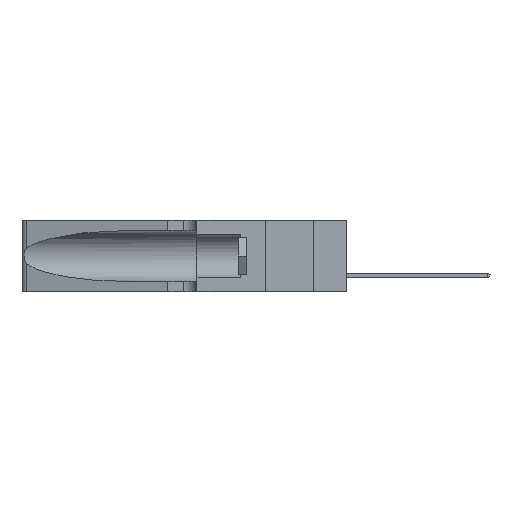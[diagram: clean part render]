
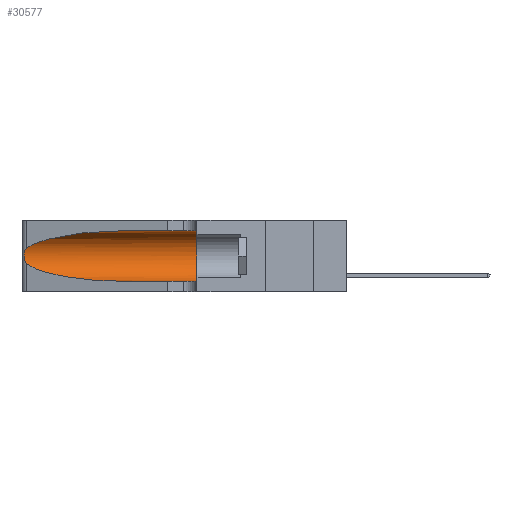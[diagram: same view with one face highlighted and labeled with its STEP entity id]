
A CAD part, left-side view. The second image highlights one B-rep face of the part: STEP entity #30577.
In plain terms, the highlighted cylindrical face has radius 3.308 mm (diameter 6.617 mm), a partial arc.
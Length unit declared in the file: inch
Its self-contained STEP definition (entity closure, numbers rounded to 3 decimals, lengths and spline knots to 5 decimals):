
#126 = CARTESIAN_POINT ( 'NONE',  ( 0.2373, 1.15595, 0.28018 ) ) ;
#372 = VERTEX_POINT ( 'NONE', #4743 ) ;
#476 = CARTESIAN_POINT ( 'NONE',  ( 0.1305, 1.61858, 0.05475 ) ) ;
#1925 = EDGE_CURVE ( 'NONE', #12517, #10170, #16900, .T. ) ;
#2455 = CARTESIAN_POINT ( 'NONE',  ( 0.18966, 0.96281, 0.31525 ) ) ;
#2658 = CARTESIAN_POINT ( 'NONE',  ( 0.25487, 1.22718, 0.22369 ) ) ;
#3737 = CARTESIAN_POINT ( 'NONE',  ( 0.25639, 1.23186, 0.15144 ) ) ;
#4407 = DIRECTION ( 'NONE',  ( 0., -1., 0. ) ) ;
#4561 = CARTESIAN_POINT ( 'NONE',  ( 0.1305, 0.72297, 0.05475 ) ) ;
#4666 = CARTESIAN_POINT ( 'NONE',  ( 0.2373, 1.15595, 0.08982 ) ) ;
#4743 = CARTESIAN_POINT ( 'NONE',  ( 0.1305, 0.72297, 0.05475 ) ) ;
#5673 = CARTESIAN_POINT ( 'NONE',  ( 0.1305, 0.35, 0.31525 ) ) ;
#6467 = CARTESIAN_POINT ( 'NONE',  ( 0.25787, 1.23484, 0.2124 ) ) ;
#6746 = CARTESIAN_POINT ( 'NONE',  ( 0.25487, 1.22718, 0.14631 ) ) ;
#7070 = VECTOR ( 'NONE', #4407, 39.37008 ) ;
#7415 = EDGE_LOOP ( 'NONE', ( #31321, #10842, #28997, #7522, #29710, #15235 ) ) ;
#7522 = ORIENTED_EDGE ( 'NONE', *, *, #19488, .T. ) ;
#9428 = DIRECTION ( 'NONE',  ( 0., 0., 1. ) ) ;
#9663 = B_SPLINE_CURVE_WITH_KNOTS ( 'NONE', 3,
 ( #26254, #21029, #13713, #6467, #28446, #13601, #28564, #31254, #15988, #25930, #18740, #3737, #12829, #10019 ),
 .UNSPECIFIED., .F., .F.,
 ( 4, 2, 2, 2, 2, 2, 4 ),
 ( 0., 0.00027, 0.00053, 0.00107, 0.0016, 0.00187, 0.00214 ),
 .UNSPECIFIED. ) ;
#10004 = CARTESIAN_POINT ( 'NONE',  ( 0.1305, 0.72297, 0.31525 ) ) ;
#10019 = CARTESIAN_POINT ( 'NONE',  ( 0.25487, 1.22718, 0.14631 ) ) ;
#10170 = VERTEX_POINT ( 'NONE', #15885 ) ;
#10484 = VERTEX_POINT ( 'NONE', #26827 ) ;
#10842 = ORIENTED_EDGE ( 'NONE', *, *, #18604, .T. ) ;
#11501 = FACE_OUTER_BOUND ( 'NONE', #7415, .T. ) ;
#12455 = DIRECTION ( 'NONE',  ( 0., 0., -1. ) ) ;
#12517 = VERTEX_POINT ( 'NONE', #18725 ) ;
#12518 = LINE ( 'NONE', #17105, #7070 ) ;
#12829 = CARTESIAN_POINT ( 'NONE',  ( 0.25555, 1.22993, 0.14849 ) ) ;
#13601 = CARTESIAN_POINT ( 'NONE',  ( 0.26018, 1.23835, 0.19895 ) ) ;
#13713 = CARTESIAN_POINT ( 'NONE',  ( 0.25639, 1.23184, 0.21858 ) ) ;
#14036 = CARTESIAN_POINT ( 'NONE',  ( 0.1305, 0.35, 0.185 ) ) ;
#14392 = LINE ( 'NONE', #476, #31277 ) ;
#14601 = DIRECTION ( 'NONE',  ( 0., -1., 0. ) ) ;
#14687 = EDGE_CURVE ( 'NONE', #12517, #25690, #12518, .T. ) ;
#15202 = CARTESIAN_POINT ( 'NONE',  ( 0.1305, 1.61858, 0.185 ) ) ;
#15235 = ORIENTED_EDGE ( 'NONE', *, *, #14687, .F. ) ;
#15885 = CARTESIAN_POINT ( 'NONE',  ( 0.25487, 1.22718, 0.22369 ) ) ;
#15988 = CARTESIAN_POINT ( 'NONE',  ( 0.26017, 1.23833, 0.17102 ) ) ;
#16491 = AXIS2_PLACEMENT_3D ( 'NONE', #15202, #14601, #12455 ) ;
#16744 = EDGE_CURVE ( 'NONE', #25690, #10484, #16775, .T. ) ;
#16775 = CIRCLE ( 'NONE', #18930, 0.13025 ) ;
#16900 =( BOUNDED_CURVE ( )  B_SPLINE_CURVE ( 3, ( #10004, #2455, #126, #2658 ),
 .UNSPECIFIED., .F., .F. ) 
 B_SPLINE_CURVE_WITH_KNOTS ( ( 4, 4 ),
 ( 1.5708, 2.84003 ),
 .UNSPECIFIED. ) 
 CURVE ( )  GEOMETRIC_REPRESENTATION_ITEM ( )  RATIONAL_B_SPLINE_CURVE ( ( 1., 0.87, 0.87, 1. ) ) 
 REPRESENTATION_ITEM ( '' )  );
#17105 = CARTESIAN_POINT ( 'NONE',  ( 0.1305, 1.61858, 0.31525 ) ) ;
#18365 = DIRECTION ( 'NONE',  ( 0., -1., 0. ) ) ;
#18604 = EDGE_CURVE ( 'NONE', #10170, #19517, #9663, .T. ) ;
#18725 = CARTESIAN_POINT ( 'NONE',  ( 0.1305, 0.72297, 0.31525 ) ) ;
#18740 = CARTESIAN_POINT ( 'NONE',  ( 0.25789, 1.23486, 0.15765 ) ) ;
#18930 = AXIS2_PLACEMENT_3D ( 'NONE', #14036, #29018, #9428 ) ;
#19488 = EDGE_CURVE ( 'NONE', #372, #10484, #14392, .T. ) ;
#19517 = VERTEX_POINT ( 'NONE', #6746 ) ;
#21029 = CARTESIAN_POINT ( 'NONE',  ( 0.25555, 1.22994, 0.2215 ) ) ;
#22209 = CARTESIAN_POINT ( 'NONE',  ( 0.18966, 0.96281, 0.05475 ) ) ;
#24476 = CARTESIAN_POINT ( 'NONE',  ( 0.25487, 1.22718, 0.14631 ) ) ;
#25690 = VERTEX_POINT ( 'NONE', #5673 ) ;
#25930 = CARTESIAN_POINT ( 'NONE',  ( 0.25856, 1.23593, 0.16098 ) ) ;
#26254 = CARTESIAN_POINT ( 'NONE',  ( 0.25487, 1.22718, 0.22369 ) ) ;
#26827 = CARTESIAN_POINT ( 'NONE',  ( 0.1305, 0.35, 0.05475 ) ) ;
#27448 = EDGE_CURVE ( 'NONE', #19517, #372, #31394, .T. ) ;
#28446 = CARTESIAN_POINT ( 'NONE',  ( 0.25854, 1.2359, 0.20912 ) ) ;
#28564 = CARTESIAN_POINT ( 'NONE',  ( 0.26075, 1.23896, 0.19203 ) ) ;
#28997 = ORIENTED_EDGE ( 'NONE', *, *, #27448, .T. ) ;
#29018 = DIRECTION ( 'NONE',  ( 0., 1., 0. ) ) ;
#29710 = ORIENTED_EDGE ( 'NONE', *, *, #16744, .F. ) ;
#30577 = ADVANCED_FACE ( 'NONE', ( #11501 ), #30713, .F. ) ;
#30713 = CYLINDRICAL_SURFACE ( 'NONE', #16491, 0.13025 ) ;
#31254 = CARTESIAN_POINT ( 'NONE',  ( 0.26075, 1.23896, 0.178 ) ) ;
#31277 = VECTOR ( 'NONE', #18365, 39.37008 ) ;
#31321 = ORIENTED_EDGE ( 'NONE', *, *, #1925, .T. ) ;
#31394 =( BOUNDED_CURVE ( )  B_SPLINE_CURVE ( 3, ( #24476, #4666, #22209, #4561 ),
 .UNSPECIFIED., .F., .F. ) 
 B_SPLINE_CURVE_WITH_KNOTS ( ( 4, 4 ),
 ( 3.44316, 4.71239 ),
 .UNSPECIFIED. ) 
 CURVE ( )  GEOMETRIC_REPRESENTATION_ITEM ( )  RATIONAL_B_SPLINE_CURVE ( ( 1., 0.87, 0.87, 1. ) ) 
 REPRESENTATION_ITEM ( '' )  );
